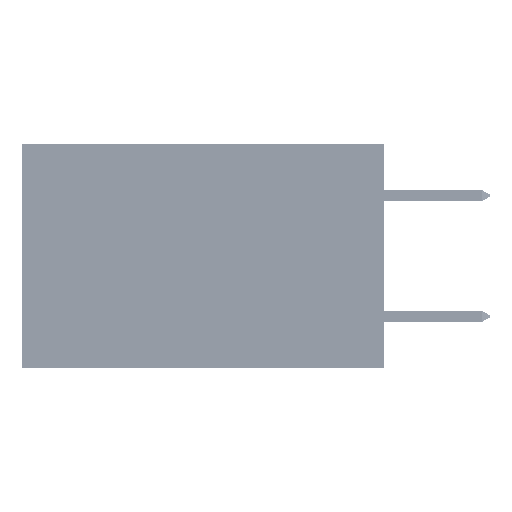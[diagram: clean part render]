
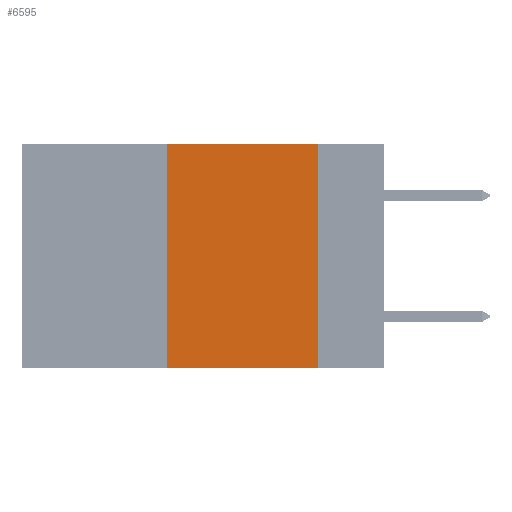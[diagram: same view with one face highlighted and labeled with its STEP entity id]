
A CAD part, left-side view. The second image highlights one B-rep face of the part: STEP entity #6595.
In plain terms, the highlighted planar face has unit normal (-1, 0, 0).
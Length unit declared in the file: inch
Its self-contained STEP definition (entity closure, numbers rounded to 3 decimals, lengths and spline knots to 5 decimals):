
#117 = CARTESIAN_POINT ( 'NONE',  ( 0., 0.6, 0. ) ) ;
#533 = ORIENTED_EDGE ( 'NONE', *, *, #24832, .F. ) ;
#1270 = VECTOR ( 'NONE', #38905, 39.37008 ) ;
#2025 = VERTEX_POINT ( 'NONE', #28222 ) ;
#4106 = PLANE ( 'NONE',  #7589 ) ;
#4355 = LINE ( 'NONE', #14844, #1270 ) ;
#5979 = CARTESIAN_POINT ( 'NONE',  ( 0., 0.36, 0. ) ) ;
#6595 = ADVANCED_FACE ( 'NONE', ( #23674 ), #4106, .F. ) ;
#7589 = AXIS2_PLACEMENT_3D ( 'NONE', #117, #35574, #27622 ) ;
#11692 = EDGE_CURVE ( 'NONE', #40270, #34581, #12213, .T. ) ;
#11711 = CARTESIAN_POINT ( 'NONE',  ( 0., 0.36, 0. ) ) ;
#12213 = LINE ( 'NONE', #20518, #37577 ) ;
#12385 = DIRECTION ( 'NONE',  ( 0., -1., 0. ) ) ;
#14844 = CARTESIAN_POINT ( 'NONE',  ( 0., 0.11, 0. ) ) ;
#16894 = VECTOR ( 'NONE', #12385, 39.37008 ) ;
#20518 = CARTESIAN_POINT ( 'NONE',  ( 0., 0.6, 0. ) ) ;
#22934 = DIRECTION ( 'NONE',  ( 0., 0., 1. ) ) ;
#23674 = FACE_OUTER_BOUND ( 'NONE', #33977, .T. ) ;
#24221 = ORIENTED_EDGE ( 'NONE', *, *, #11692, .F. ) ;
#24481 = DIRECTION ( 'NONE',  ( 0., -1., 0. ) ) ;
#24832 = EDGE_CURVE ( 'NONE', #34581, #25924, #4355, .T. ) ;
#25924 = VERTEX_POINT ( 'NONE', #29555 ) ;
#27622 = DIRECTION ( 'NONE',  ( 0., 0., -1. ) ) ;
#28222 = CARTESIAN_POINT ( 'NONE',  ( 0., 0.36, -0.37 ) ) ;
#29545 = EDGE_CURVE ( 'NONE', #2025, #40270, #35864, .T. ) ;
#29555 = CARTESIAN_POINT ( 'NONE',  ( 0., 0.11, -0.37 ) ) ;
#33656 = LINE ( 'NONE', #36064, #16894 ) ;
#33977 = EDGE_LOOP ( 'NONE', ( #533, #24221, #43879, #40064 ) ) ;
#34472 = EDGE_CURVE ( 'NONE', #2025, #25924, #33656, .T. ) ;
#34581 = VERTEX_POINT ( 'NONE', #48886 ) ;
#35574 = DIRECTION ( 'NONE',  ( 1., 0., 0. ) ) ;
#35864 = LINE ( 'NONE', #11711, #41486 ) ;
#36064 = CARTESIAN_POINT ( 'NONE',  ( 0., 0.6, -0.37 ) ) ;
#37577 = VECTOR ( 'NONE', #24481, 39.37008 ) ;
#38905 = DIRECTION ( 'NONE',  ( 0., 0., -1. ) ) ;
#40064 = ORIENTED_EDGE ( 'NONE', *, *, #34472, .T. ) ;
#40270 = VERTEX_POINT ( 'NONE', #5979 ) ;
#41486 = VECTOR ( 'NONE', #22934, 39.37008 ) ;
#43879 = ORIENTED_EDGE ( 'NONE', *, *, #29545, .F. ) ;
#48886 = CARTESIAN_POINT ( 'NONE',  ( 0., 0.11, 0. ) ) ;
